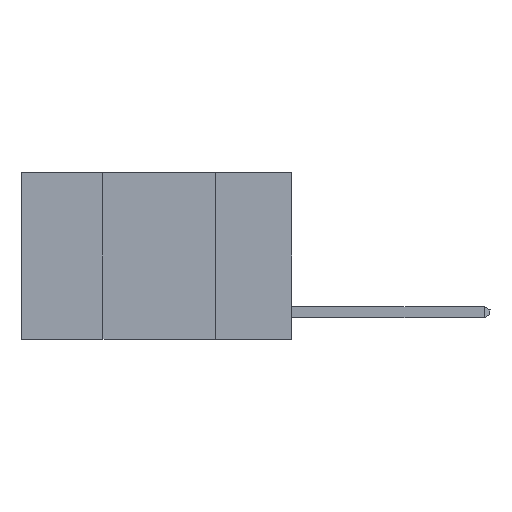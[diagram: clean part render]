
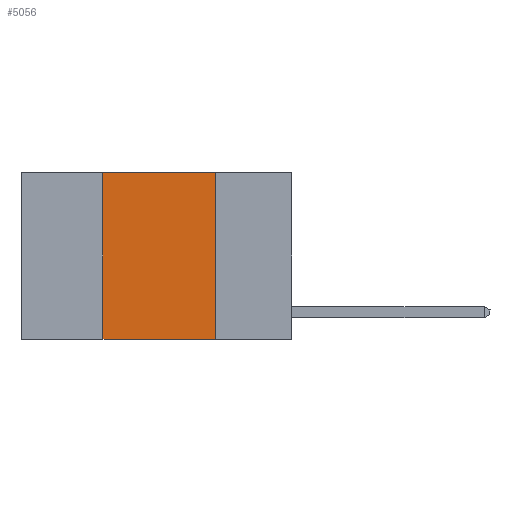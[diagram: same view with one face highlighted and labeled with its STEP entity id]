
A CAD part, left-side view. The second image highlights one B-rep face of the part: STEP entity #5056.
In plain terms, the highlighted planar face has unit normal (-1, 0, 0).
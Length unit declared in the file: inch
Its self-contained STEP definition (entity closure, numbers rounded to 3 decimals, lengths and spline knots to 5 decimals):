
#144 = CARTESIAN_POINT ( 'NONE',  ( 0., 0.6, -0.37 ) ) ;
#230 = ORIENTED_EDGE ( 'NONE', *, *, #9558, .T. ) ;
#481 = VERTEX_POINT ( 'NONE', #7488 ) ;
#743 = VERTEX_POINT ( 'NONE', #1994 ) ;
#1147 = CARTESIAN_POINT ( 'NONE',  ( 0., 0.42, 0. ) ) ;
#1248 = EDGE_CURVE ( 'NONE', #14965, #481, #8707, .T. ) ;
#1707 = EDGE_CURVE ( 'NONE', #2185, #14965, #5623, .T. ) ;
#1735 = LINE ( 'NONE', #144, #7971 ) ;
#1994 = CARTESIAN_POINT ( 'NONE',  ( 0., 0.42, -0.37 ) ) ;
#2185 = VERTEX_POINT ( 'NONE', #4870 ) ;
#2218 = CARTESIAN_POINT ( 'NONE',  ( 0., 0.6, 0. ) ) ;
#3344 = ORIENTED_EDGE ( 'NONE', *, *, #4400, .F. ) ;
#3621 = PLANE ( 'NONE',  #11142 ) ;
#4400 = EDGE_CURVE ( 'NONE', #743, #2185, #16007, .T. ) ;
#4730 = DIRECTION ( 'NONE',  ( 0., -1., 0. ) ) ;
#4870 = CARTESIAN_POINT ( 'NONE',  ( 0., 0.42, 0. ) ) ;
#4883 = DIRECTION ( 'NONE',  ( 0., 0., -1. ) ) ;
#5056 = ADVANCED_FACE ( 'NONE', ( #12894 ), #3621, .F. ) ;
#5623 = LINE ( 'NONE', #2218, #11757 ) ;
#6248 = CARTESIAN_POINT ( 'NONE',  ( 0., 0.17, 0. ) ) ;
#7488 = CARTESIAN_POINT ( 'NONE',  ( 0., 0.17, -0.37 ) ) ;
#7825 = DIRECTION ( 'NONE',  ( 0., 0., -1. ) ) ;
#7971 = VECTOR ( 'NONE', #9067, 39.37008 ) ;
#8047 = CARTESIAN_POINT ( 'NONE',  ( 0., 0.17, 0. ) ) ;
#8546 = CARTESIAN_POINT ( 'NONE',  ( 0., 0.6, 0. ) ) ;
#8664 = DIRECTION ( 'NONE',  ( 0., 0., 1. ) ) ;
#8707 = LINE ( 'NONE', #6248, #15275 ) ;
#8745 = ORIENTED_EDGE ( 'NONE', *, *, #1248, .F. ) ;
#9003 = EDGE_LOOP ( 'NONE', ( #8745, #9142, #3344, #230 ) ) ;
#9067 = DIRECTION ( 'NONE',  ( 0., -1., 0. ) ) ;
#9142 = ORIENTED_EDGE ( 'NONE', *, *, #1707, .F. ) ;
#9558 = EDGE_CURVE ( 'NONE', #743, #481, #1735, .T. ) ;
#11142 = AXIS2_PLACEMENT_3D ( 'NONE', #8546, #12235, #4883 ) ;
#11757 = VECTOR ( 'NONE', #4730, 39.37008 ) ;
#12235 = DIRECTION ( 'NONE',  ( 1., 0., 0. ) ) ;
#12894 = FACE_OUTER_BOUND ( 'NONE', #9003, .T. ) ;
#14965 = VERTEX_POINT ( 'NONE', #8047 ) ;
#15247 = VECTOR ( 'NONE', #8664, 39.37008 ) ;
#15275 = VECTOR ( 'NONE', #7825, 39.37008 ) ;
#16007 = LINE ( 'NONE', #1147, #15247 ) ;
